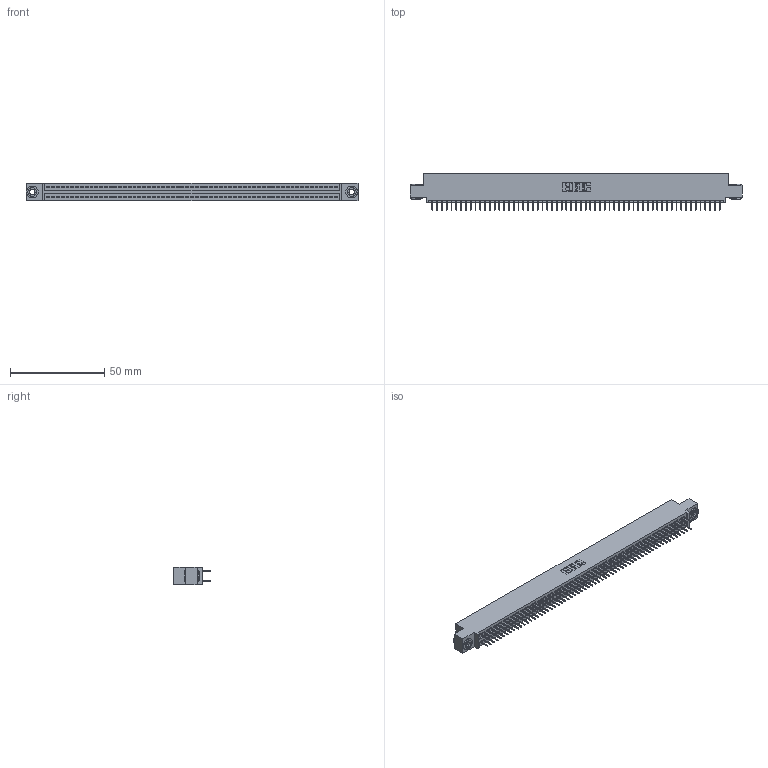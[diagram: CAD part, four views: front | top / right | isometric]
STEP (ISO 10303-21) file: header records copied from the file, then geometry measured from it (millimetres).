
FILE_DESCRIPTION (( 'STEP AP203' ), '1' );
FILE_NAME ('395-122-524-503.STEP', '2018-12-03T17:37:58', ( '' ), ( '' ), 'SwSTEP 2.0', 'SolidWorks 2016', '' );
FILE_SCHEMA (( 'CONFIG_CONTROL_DESIGN' ));
Length unit declared in the file: inch
Products named in the file (4): 395-122-524-503; 345 Part_0.110 Offset - 0.156 Dia-TH; 345-250-002_345-250-002-102; 345-292-001_345-293-124
Assembly tree (125 placements, depth 2):
  395-122-524-503
    345 Part_0.110 Offset - 0.156 Dia-TH
    345-292-001_345-293-124  x122
    345-250-002_345-250-002-102  x2
Bounding box: 176.15 x 19.35 x 9.4 mm (x, y, z)
Volume: 17049.1 mm3; surface area: 25379.7 mm2
Topology: 125 solids, 125 shells, 6756 faces, 19095 edges, 12238 vertices
Faces by surface type: plane 4852, cylinder 1896, cone 8
Entity records: 46160 total; most frequent: CARTESIAN_POINT 7695, ORIENTED_EDGE 7622, DIRECTION 6793, EDGE_CURVE 3811, LINE 3415, VECTOR 3415, VERTEX_POINT 2534, AXIS2_PLACEMENT_3D 1689
